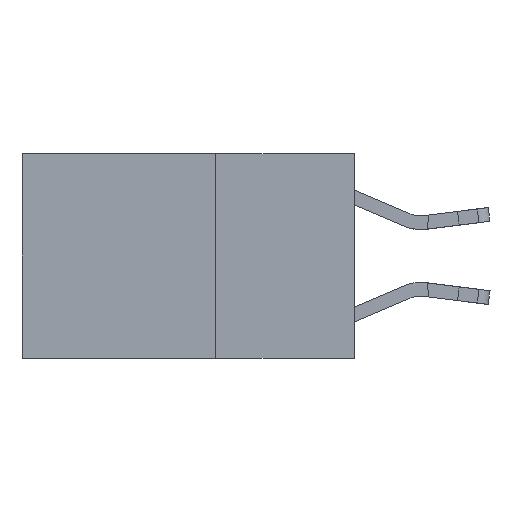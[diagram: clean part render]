
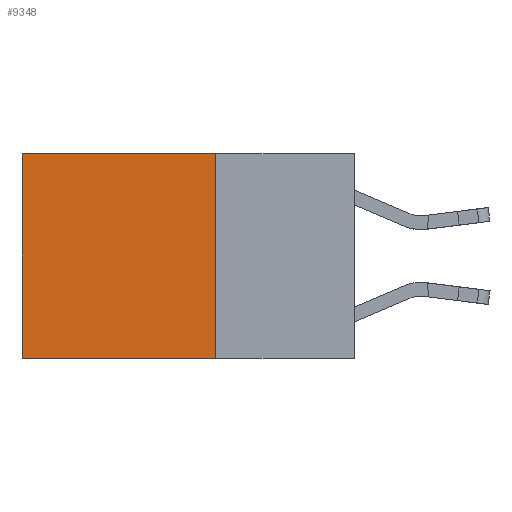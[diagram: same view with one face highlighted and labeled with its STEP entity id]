
A CAD part, left-side view. The second image highlights one B-rep face of the part: STEP entity #9348.
In plain terms, the highlighted planar face has unit normal (-1, 0, 0).
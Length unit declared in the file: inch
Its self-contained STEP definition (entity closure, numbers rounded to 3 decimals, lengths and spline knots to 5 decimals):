
#1017 = CARTESIAN_POINT ( 'NONE',  ( 0.2625, 0.25, 0. ) ) ;
#1159 = CARTESIAN_POINT ( 'NONE',  ( 0.2625, 0.25, -0.37 ) ) ;
#2018 = CARTESIAN_POINT ( 'NONE',  ( 0.2625, 0.25, -0.37 ) ) ;
#2689 = ORIENTED_EDGE ( 'NONE', *, *, #4538, .F. ) ;
#3708 = VECTOR ( 'NONE', #7796, 39.37008 ) ;
#4339 = VECTOR ( 'NONE', #13630, 39.37008 ) ;
#4538 = EDGE_CURVE ( 'NONE', #18925, #13587, #21878, .T. ) ;
#4601 = VECTOR ( 'NONE', #7118, 39.37008 ) ;
#5153 = LINE ( 'NONE', #17835, #4601 ) ;
#5832 = AXIS2_PLACEMENT_3D ( 'NONE', #17344, #22750, #19285 ) ;
#6410 = ORIENTED_EDGE ( 'NONE', *, *, #7390, .T. ) ;
#6977 = ORIENTED_EDGE ( 'NONE', *, *, #10207, .T. ) ;
#7118 = DIRECTION ( 'NONE',  ( 0., 1., 0. ) ) ;
#7390 = EDGE_CURVE ( 'NONE', #19674, #13587, #16203, .T. ) ;
#7796 = DIRECTION ( 'NONE',  ( 0., 0., -1. ) ) ;
#8493 = PLANE ( 'NONE',  #5832 ) ;
#8741 = CARTESIAN_POINT ( 'NONE',  ( 0.2625, 0.6, 0. ) ) ;
#9348 = ADVANCED_FACE ( 'NONE', ( #11081 ), #8493, .F. ) ;
#10207 = EDGE_CURVE ( 'NONE', #14748, #19674, #5153, .T. ) ;
#11081 = FACE_OUTER_BOUND ( 'NONE', #12709, .T. ) ;
#12709 = EDGE_LOOP ( 'NONE', ( #6410, #2689, #21622, #6977 ) ) ;
#13587 = VERTEX_POINT ( 'NONE', #21979 ) ;
#13630 = DIRECTION ( 'NONE',  ( 0., 1., 0. ) ) ;
#14748 = VERTEX_POINT ( 'NONE', #21113 ) ;
#15384 = DIRECTION ( 'NONE',  ( 0., 0., -1. ) ) ;
#16203 = LINE ( 'NONE', #17000, #3708 ) ;
#17000 = CARTESIAN_POINT ( 'NONE',  ( 0.2625, 0.6, 0. ) ) ;
#17344 = CARTESIAN_POINT ( 'NONE',  ( 0.2625, 0.25, 0. ) ) ;
#17835 = CARTESIAN_POINT ( 'NONE',  ( 0.2625, 0.25, 0. ) ) ;
#18726 = VECTOR ( 'NONE', #15384, 39.37008 ) ;
#18925 = VERTEX_POINT ( 'NONE', #2018 ) ;
#19285 = DIRECTION ( 'NONE',  ( 0., 0., -1. ) ) ;
#19674 = VERTEX_POINT ( 'NONE', #8741 ) ;
#20307 = EDGE_CURVE ( 'NONE', #14748, #18925, #22627, .T. ) ;
#21113 = CARTESIAN_POINT ( 'NONE',  ( 0.2625, 0.25, 0. ) ) ;
#21622 = ORIENTED_EDGE ( 'NONE', *, *, #20307, .F. ) ;
#21878 = LINE ( 'NONE', #1159, #4339 ) ;
#21979 = CARTESIAN_POINT ( 'NONE',  ( 0.2625, 0.6, -0.37 ) ) ;
#22627 = LINE ( 'NONE', #1017, #18726 ) ;
#22750 = DIRECTION ( 'NONE',  ( 1., 0., 0. ) ) ;
